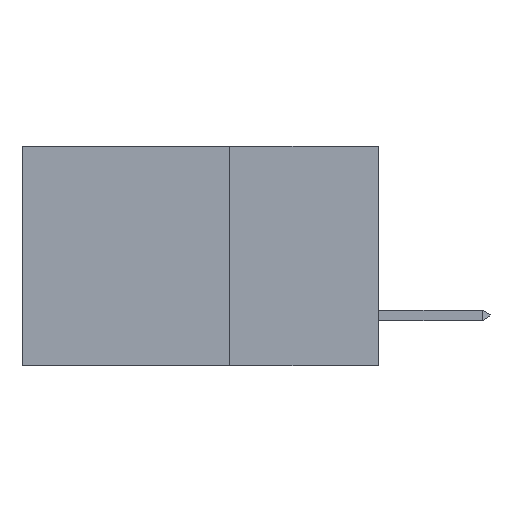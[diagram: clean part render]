
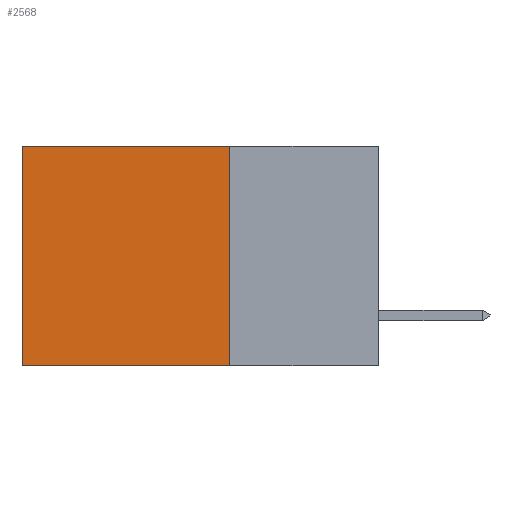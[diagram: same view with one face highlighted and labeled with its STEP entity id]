
A CAD part, left-side view. The second image highlights one B-rep face of the part: STEP entity #2568.
In plain terms, the highlighted planar face has unit normal (-1, 0, 0).
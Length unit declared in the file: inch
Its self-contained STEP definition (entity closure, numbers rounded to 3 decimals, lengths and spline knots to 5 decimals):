
#344 = LINE ( 'NONE', #7521, #5804 ) ;
#764 = DIRECTION ( 'NONE',  ( 0., 1., 0. ) ) ;
#812 = EDGE_CURVE ( 'NONE', #10572, #3587, #958, .T. ) ;
#958 = LINE ( 'NONE', #10938, #5132 ) ;
#2224 = ORIENTED_EDGE ( 'NONE', *, *, #812, .T. ) ;
#2568 = ADVANCED_FACE ( 'NONE', ( #12457 ), #3589, .F. ) ;
#2734 = VECTOR ( 'NONE', #12424, 39.37008 ) ;
#2793 = DIRECTION ( 'NONE',  ( 1., 0., 0. ) ) ;
#2840 = EDGE_CURVE ( 'NONE', #10664, #12341, #344, .T. ) ;
#3251 = CARTESIAN_POINT ( 'NONE',  ( 0.2615, 0.25, -0.37 ) ) ;
#3584 = ORIENTED_EDGE ( 'NONE', *, *, #2840, .F. ) ;
#3587 = VERTEX_POINT ( 'NONE', #12744 ) ;
#3589 = PLANE ( 'NONE',  #10970 ) ;
#5132 = VECTOR ( 'NONE', #12764, 39.37008 ) ;
#5227 = EDGE_CURVE ( 'NONE', #10664, #10572, #8541, .T. ) ;
#5804 = VECTOR ( 'NONE', #8483, 39.37008 ) ;
#6757 = DIRECTION ( 'NONE',  ( 0., 0., -1. ) ) ;
#6821 = CARTESIAN_POINT ( 'NONE',  ( 0.2615, 0.25, -0.37 ) ) ;
#6883 = CARTESIAN_POINT ( 'NONE',  ( 0.2615, 0.25, -0.37 ) ) ;
#7521 = CARTESIAN_POINT ( 'NONE',  ( 0.2615, 0.25, -0.37 ) ) ;
#8151 = ORIENTED_EDGE ( 'NONE', *, *, #5227, .T. ) ;
#8364 = LINE ( 'NONE', #3251, #12013 ) ;
#8483 = DIRECTION ( 'NONE',  ( 0., 0., -1. ) ) ;
#8541 = LINE ( 'NONE', #9715, #2734 ) ;
#9478 = EDGE_LOOP ( 'NONE', ( #2224, #11364, #3584, #8151 ) ) ;
#9561 = EDGE_CURVE ( 'NONE', #12341, #3587, #8364, .T. ) ;
#9715 = CARTESIAN_POINT ( 'NONE',  ( 0.2615, 0.25, 0. ) ) ;
#10572 = VERTEX_POINT ( 'NONE', #11802 ) ;
#10664 = VERTEX_POINT ( 'NONE', #11609 ) ;
#10938 = CARTESIAN_POINT ( 'NONE',  ( 0.2615, 0.6, -0.37 ) ) ;
#10970 = AXIS2_PLACEMENT_3D ( 'NONE', #6821, #2793, #6757 ) ;
#11364 = ORIENTED_EDGE ( 'NONE', *, *, #9561, .F. ) ;
#11609 = CARTESIAN_POINT ( 'NONE',  ( 0.2615, 0.25, 0. ) ) ;
#11802 = CARTESIAN_POINT ( 'NONE',  ( 0.2615, 0.6, 0. ) ) ;
#12013 = VECTOR ( 'NONE', #764, 39.37008 ) ;
#12341 = VERTEX_POINT ( 'NONE', #6883 ) ;
#12424 = DIRECTION ( 'NONE',  ( 0., 1., 0. ) ) ;
#12457 = FACE_OUTER_BOUND ( 'NONE', #9478, .T. ) ;
#12744 = CARTESIAN_POINT ( 'NONE',  ( 0.2615, 0.6, -0.37 ) ) ;
#12764 = DIRECTION ( 'NONE',  ( 0., 0., -1. ) ) ;
